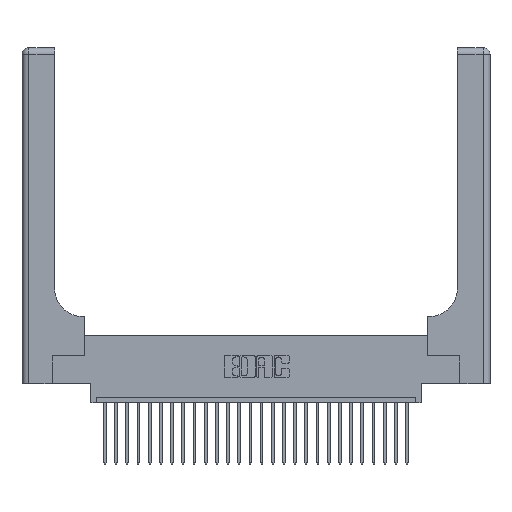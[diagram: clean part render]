
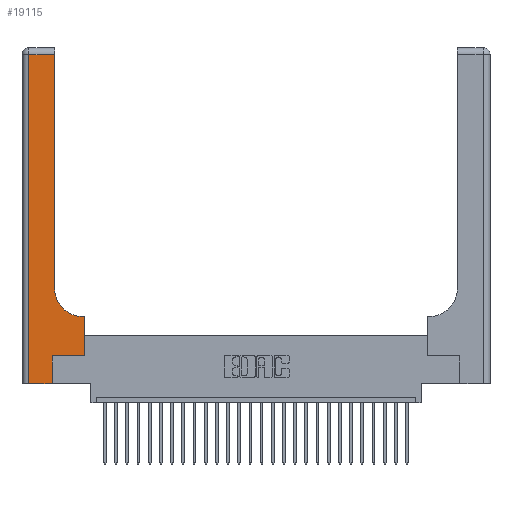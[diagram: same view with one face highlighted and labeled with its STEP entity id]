
A CAD part, top view. The second image highlights one B-rep face of the part: STEP entity #19115.
In plain terms, the highlighted planar face has unit normal (0, 0, 1).
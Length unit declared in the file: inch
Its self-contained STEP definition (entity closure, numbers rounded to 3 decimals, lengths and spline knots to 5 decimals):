
#1309 = CARTESIAN_POINT ( 'NONE',  ( 0.5585, 0.25, 0.37 ) ) ;
#1417 = DIRECTION ( 'NONE',  ( 0., 1., 0. ) ) ;
#1514 = CARTESIAN_POINT ( 'NONE',  ( 0.269, 0., 0.37 ) ) ;
#2077 = DIRECTION ( 'NONE',  ( -1., 0., 0. ) ) ;
#2663 = AXIS2_PLACEMENT_3D ( 'NONE', #17599, #26369, #10822 ) ;
#3443 = CARTESIAN_POINT ( 'NONE',  ( 0.269, 0.25, 0.37 ) ) ;
#3789 = DIRECTION ( 'NONE',  ( 0., -1., 0. ) ) ;
#4373 = FACE_OUTER_BOUND ( 'NONE', #20982, .T. ) ;
#4583 = VECTOR ( 'NONE', #3789, 39.37008 ) ;
#4688 = VECTOR ( 'NONE', #22655, 39.37008 ) ;
#4735 = EDGE_CURVE ( 'NONE', #8073, #6195, #13602, .T. ) ;
#5311 = AXIS2_PLACEMENT_3D ( 'NONE', #27801, #10236, #21143 ) ;
#5403 = CARTESIAN_POINT ( 'NONE',  ( 0.269, 0., 0.37 ) ) ;
#5461 = EDGE_CURVE ( 'NONE', #15839, #22997, #17348, .T. ) ;
#5803 = ORIENTED_EDGE ( 'NONE', *, *, #21893, .T. ) ;
#6195 = VERTEX_POINT ( 'NONE', #3443 ) ;
#6821 = CARTESIAN_POINT ( 'NONE',  ( 0.269, 0.25, 0.37 ) ) ;
#7384 = EDGE_CURVE ( 'NONE', #6195, #15839, #13813, .T. ) ;
#7566 = ORIENTED_EDGE ( 'NONE', *, *, #20125, .T. ) ;
#8073 = VERTEX_POINT ( 'NONE', #1514 ) ;
#9051 = EDGE_CURVE ( 'NONE', #11490, #17306, #24892, .T. ) ;
#9718 = DIRECTION ( 'NONE',  ( 0., 1., 0. ) ) ;
#10236 = DIRECTION ( 'NONE',  ( 0., 0., -1. ) ) ;
#10412 = VECTOR ( 'NONE', #13897, 39.37008 ) ;
#10822 = DIRECTION ( 'NONE',  ( -1., 0., 0. ) ) ;
#11153 = LINE ( 'NONE', #23762, #28251 ) ;
#11474 = ORIENTED_EDGE ( 'NONE', *, *, #7384, .T. ) ;
#11490 = VERTEX_POINT ( 'NONE', #18311 ) ;
#11522 = LINE ( 'NONE', #26568, #25903 ) ;
#12067 = VERTEX_POINT ( 'NONE', #19135 ) ;
#12663 = CARTESIAN_POINT ( 'NONE',  ( 0.06, 2.94, 0.37 ) ) ;
#13011 = PLANE ( 'NONE',  #2663 ) ;
#13602 = LINE ( 'NONE', #5403, #20791 ) ;
#13609 = VECTOR ( 'NONE', #1417, 39.37008 ) ;
#13714 = DIRECTION ( 'NONE',  ( 0., 1., 0. ) ) ;
#13813 = LINE ( 'NONE', #6821, #10412 ) ;
#13897 = DIRECTION ( 'NONE',  ( 1., 0., 0. ) ) ;
#14197 = VERTEX_POINT ( 'NONE', #24315 ) ;
#14271 = LINE ( 'NONE', #26947, #4688 ) ;
#14488 = CARTESIAN_POINT ( 'NONE',  ( 0.2915, 3., 0.37 ) ) ;
#14865 = CARTESIAN_POINT ( 'NONE',  ( 0.06, 3., 0.37 ) ) ;
#15057 = ORIENTED_EDGE ( 'NONE', *, *, #23149, .T. ) ;
#15357 = CARTESIAN_POINT ( 'NONE',  ( 0.2915, 2.94, 0.37 ) ) ;
#15839 = VERTEX_POINT ( 'NONE', #22840 ) ;
#17306 = VERTEX_POINT ( 'NONE', #15357 ) ;
#17348 = LINE ( 'NONE', #1309, #28256 ) ;
#17599 = CARTESIAN_POINT ( 'NONE',  ( 0., 3., 0.37 ) ) ;
#18311 = CARTESIAN_POINT ( 'NONE',  ( 0.2915, 0.85, 0.37 ) ) ;
#18594 = CARTESIAN_POINT ( 'NONE',  ( 0.5585, 0.6, 0.37 ) ) ;
#19115 = ADVANCED_FACE ( 'NONE', ( #4373 ), #13011, .F. ) ;
#19135 = CARTESIAN_POINT ( 'NONE',  ( 0.5415, 0.6, 0.37 ) ) ;
#19774 = ORIENTED_EDGE ( 'NONE', *, *, #22048, .T. ) ;
#20040 = ORIENTED_EDGE ( 'NONE', *, *, #9051, .T. ) ;
#20125 = EDGE_CURVE ( 'NONE', #17306, #26747, #11153, .T. ) ;
#20159 = DIRECTION ( 'NONE',  ( 1., 0., 0. ) ) ;
#20791 = VECTOR ( 'NONE', #9718, 39.37008 ) ;
#20982 = EDGE_LOOP ( 'NONE', ( #20040, #7566, #15057, #26559, #22107, #11474, #26189, #5803, #19774 ) ) ;
#21143 = DIRECTION ( 'NONE',  ( 1., 0., 0. ) ) ;
#21775 = EDGE_CURVE ( 'NONE', #14197, #8073, #11522, .T. ) ;
#21893 = EDGE_CURVE ( 'NONE', #22997, #12067, #14271, .T. ) ;
#22048 = EDGE_CURVE ( 'NONE', #12067, #11490, #24829, .T. ) ;
#22107 = ORIENTED_EDGE ( 'NONE', *, *, #4735, .T. ) ;
#22655 = DIRECTION ( 'NONE',  ( -1., 0., 0. ) ) ;
#22840 = CARTESIAN_POINT ( 'NONE',  ( 0.5585, 0.25, 0.37 ) ) ;
#22997 = VERTEX_POINT ( 'NONE', #18594 ) ;
#23149 = EDGE_CURVE ( 'NONE', #26747, #14197, #25077, .T. ) ;
#23762 = CARTESIAN_POINT ( 'NONE',  ( 0., 2.94, 0.37 ) ) ;
#24315 = CARTESIAN_POINT ( 'NONE',  ( 0.06, 0., 0.37 ) ) ;
#24829 = CIRCLE ( 'NONE', #5311, 0.25 ) ;
#24892 = LINE ( 'NONE', #14488, #13609 ) ;
#25077 = LINE ( 'NONE', #14865, #4583 ) ;
#25903 = VECTOR ( 'NONE', #20159, 39.37008 ) ;
#26189 = ORIENTED_EDGE ( 'NONE', *, *, #5461, .T. ) ;
#26369 = DIRECTION ( 'NONE',  ( 0., 0., -1. ) ) ;
#26559 = ORIENTED_EDGE ( 'NONE', *, *, #21775, .T. ) ;
#26568 = CARTESIAN_POINT ( 'NONE',  ( 0., 0., 0.37 ) ) ;
#26747 = VERTEX_POINT ( 'NONE', #12663 ) ;
#26947 = CARTESIAN_POINT ( 'NONE',  ( 0.2915, 0.6, 0.37 ) ) ;
#27801 = CARTESIAN_POINT ( 'NONE',  ( 0.5415, 0.85, 0.37 ) ) ;
#28251 = VECTOR ( 'NONE', #2077, 39.37008 ) ;
#28256 = VECTOR ( 'NONE', #13714, 39.37008 ) ;
